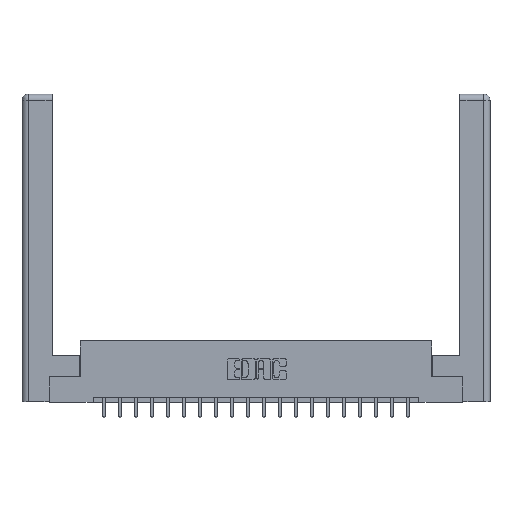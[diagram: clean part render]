
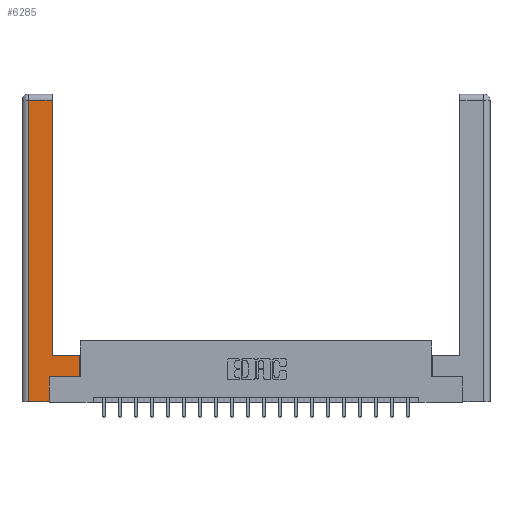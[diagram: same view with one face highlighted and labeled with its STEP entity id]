
A CAD part, top view. The second image highlights one B-rep face of the part: STEP entity #6285.
In plain terms, the highlighted planar face has unit normal (0, 0, 1).
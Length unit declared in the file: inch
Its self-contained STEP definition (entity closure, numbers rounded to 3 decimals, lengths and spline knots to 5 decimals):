
#103 = VERTEX_POINT ( 'NONE', #8155 ) ;
#119 = ORIENTED_EDGE ( 'NONE', *, *, #2896, .T. ) ;
#680 = ORIENTED_EDGE ( 'NONE', *, *, #766, .T. ) ;
#766 = EDGE_CURVE ( 'NONE', #103, #7306, #6736, .T. ) ;
#888 = ORIENTED_EDGE ( 'NONE', *, *, #17332, .T. ) ;
#919 = CARTESIAN_POINT ( 'NONE',  ( 0.0615, 0., 0. ) ) ;
#1154 = LINE ( 'NONE', #20083, #9099 ) ;
#1870 = CARTESIAN_POINT ( 'NONE',  ( 0.565, 0.45, 0. ) ) ;
#2197 = DIRECTION ( 'NONE',  ( 1., 0., 0. ) ) ;
#2314 = LINE ( 'NONE', #2506, #7186 ) ;
#2506 = CARTESIAN_POINT ( 'NONE',  ( 0.565, 0.45, 0. ) ) ;
#2896 = EDGE_CURVE ( 'NONE', #6499, #103, #11180, .T. ) ;
#3640 = ORIENTED_EDGE ( 'NONE', *, *, #5060, .T. ) ;
#4796 = VERTEX_POINT ( 'NONE', #1870 ) ;
#5060 = EDGE_CURVE ( 'NONE', #7306, #14530, #1154, .T. ) ;
#5500 = ORIENTED_EDGE ( 'NONE', *, *, #13719, .T. ) ;
#5576 = LINE ( 'NONE', #11341, #16241 ) ;
#5651 = CARTESIAN_POINT ( 'NONE',  ( 0., 0., 0. ) ) ;
#6280 = FACE_OUTER_BOUND ( 'NONE', #14070, .T. ) ;
#6285 = ADVANCED_FACE ( 'NONE', ( #6280 ), #15458, .F. ) ;
#6499 = VERTEX_POINT ( 'NONE', #9372 ) ;
#6736 = LINE ( 'NONE', #11567, #16129 ) ;
#6861 = VERTEX_POINT ( 'NONE', #19837 ) ;
#6869 = CARTESIAN_POINT ( 'NONE',  ( 0.265, 0., 0. ) ) ;
#6909 = LINE ( 'NONE', #7948, #15298 ) ;
#7186 = VECTOR ( 'NONE', #7796, 39.37008 ) ;
#7306 = VERTEX_POINT ( 'NONE', #11454 ) ;
#7675 = CARTESIAN_POINT ( 'NONE',  ( 0.295, 3., 0. ) ) ;
#7777 = LINE ( 'NONE', #18383, #17932 ) ;
#7796 = DIRECTION ( 'NONE',  ( 0., 1., 0. ) ) ;
#7948 = CARTESIAN_POINT ( 'NONE',  ( 0.265, 0., 0. ) ) ;
#8155 = CARTESIAN_POINT ( 'NONE',  ( 0.295, 2.94, 0. ) ) ;
#8958 = VECTOR ( 'NONE', #11813, 39.37008 ) ;
#9094 = ORIENTED_EDGE ( 'NONE', *, *, #11082, .T. ) ;
#9099 = VECTOR ( 'NONE', #13683, 39.37008 ) ;
#9372 = CARTESIAN_POINT ( 'NONE',  ( 0.295, 0.45, 0. ) ) ;
#9516 = DIRECTION ( 'NONE',  ( 0., 1., 0. ) ) ;
#9715 = EDGE_CURVE ( 'NONE', #6861, #4796, #2314, .T. ) ;
#9978 = CARTESIAN_POINT ( 'NONE',  ( 0.265, 0.245, 0. ) ) ;
#10369 = EDGE_CURVE ( 'NONE', #14441, #18195, #17560, .T. ) ;
#11082 = EDGE_CURVE ( 'NONE', #4796, #6499, #5576, .T. ) ;
#11180 = LINE ( 'NONE', #7675, #16268 ) ;
#11341 = CARTESIAN_POINT ( 'NONE',  ( 0.295, 0.45, 0. ) ) ;
#11454 = CARTESIAN_POINT ( 'NONE',  ( 0.0615, 2.94, 0. ) ) ;
#11567 = CARTESIAN_POINT ( 'NONE',  ( 0.0615, 2.94, 0. ) ) ;
#11813 = DIRECTION ( 'NONE',  ( 0., 1., 0. ) ) ;
#12257 = DIRECTION ( 'NONE',  ( -1., 0., 0. ) ) ;
#13382 = CARTESIAN_POINT ( 'NONE',  ( 0.265, 0.245, 0. ) ) ;
#13683 = DIRECTION ( 'NONE',  ( 0., -1., 0. ) ) ;
#13719 = EDGE_CURVE ( 'NONE', #14530, #14441, #6909, .T. ) ;
#13934 = ORIENTED_EDGE ( 'NONE', *, *, #10369, .T. ) ;
#14070 = EDGE_LOOP ( 'NONE', ( #119, #680, #3640, #5500, #13934, #888, #17685, #9094 ) ) ;
#14441 = VERTEX_POINT ( 'NONE', #6869 ) ;
#14530 = VERTEX_POINT ( 'NONE', #919 ) ;
#15298 = VECTOR ( 'NONE', #19245, 39.37008 ) ;
#15458 = PLANE ( 'NONE',  #18969 ) ;
#16019 = DIRECTION ( 'NONE',  ( -1., 0., 0. ) ) ;
#16129 = VECTOR ( 'NONE', #19607, 39.37008 ) ;
#16241 = VECTOR ( 'NONE', #16019, 39.37008 ) ;
#16268 = VECTOR ( 'NONE', #9516, 39.37008 ) ;
#17332 = EDGE_CURVE ( 'NONE', #18195, #6861, #7777, .T. ) ;
#17560 = LINE ( 'NONE', #13382, #8958 ) ;
#17685 = ORIENTED_EDGE ( 'NONE', *, *, #9715, .T. ) ;
#17932 = VECTOR ( 'NONE', #2197, 39.37008 ) ;
#18195 = VERTEX_POINT ( 'NONE', #9978 ) ;
#18383 = CARTESIAN_POINT ( 'NONE',  ( 0.565, 0.245, 0. ) ) ;
#18969 = AXIS2_PLACEMENT_3D ( 'NONE', #5651, #20356, #12257 ) ;
#19245 = DIRECTION ( 'NONE',  ( 1., 0., 0. ) ) ;
#19607 = DIRECTION ( 'NONE',  ( -1., 0., 0. ) ) ;
#19837 = CARTESIAN_POINT ( 'NONE',  ( 0.565, 0.245, 0. ) ) ;
#20083 = CARTESIAN_POINT ( 'NONE',  ( 0.0615, 0., 0. ) ) ;
#20356 = DIRECTION ( 'NONE',  ( 0., 0., -1. ) ) ;
